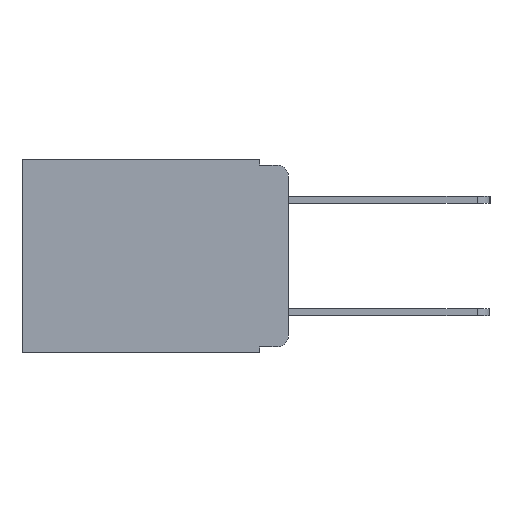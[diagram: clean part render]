
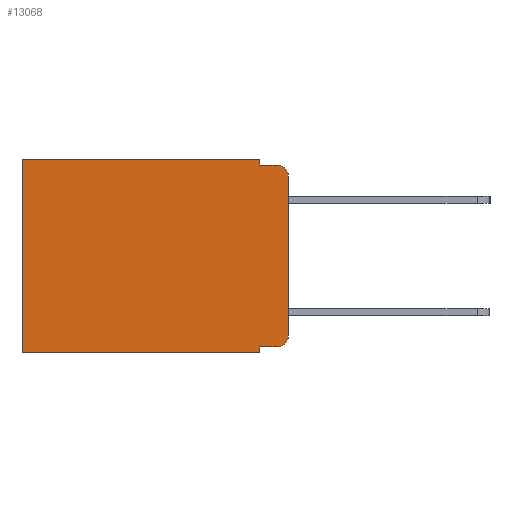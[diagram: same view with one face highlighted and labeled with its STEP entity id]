
A CAD part, left-side view. The second image highlights one B-rep face of the part: STEP entity #13068.
In plain terms, the highlighted planar face has unit normal (-1, 0, 0).
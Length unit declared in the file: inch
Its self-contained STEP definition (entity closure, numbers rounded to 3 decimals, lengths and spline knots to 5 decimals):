
#125 = DIRECTION ( 'NONE',  ( 1., 0., 0. ) ) ;
#245 = EDGE_CURVE ( 'NONE', #4848, #9189, #17565, .T. ) ;
#253 = LINE ( 'NONE', #16846, #16387 ) ;
#279 = EDGE_CURVE ( 'NONE', #9189, #9463, #1811, .T. ) ;
#335 = VERTEX_POINT ( 'NONE', #2833 ) ;
#371 = FACE_OUTER_BOUND ( 'NONE', #6724, .T. ) ;
#1110 = VERTEX_POINT ( 'NONE', #19627 ) ;
#1449 = ORIENTED_EDGE ( 'NONE', *, *, #13762, .F. ) ;
#1811 = CIRCLE ( 'NONE', #2198, 0.02 ) ;
#2198 = AXIS2_PLACEMENT_3D ( 'NONE', #12227, #4207, #6741 ) ;
#2668 = ORIENTED_EDGE ( 'NONE', *, *, #245, .T. ) ;
#2699 = VERTEX_POINT ( 'NONE', #14720 ) ;
#2833 = CARTESIAN_POINT ( 'NONE',  ( 0.298, 0.473, -0.343 ) ) ;
#3286 = EDGE_CURVE ( 'NONE', #2699, #335, #19096, .T. ) ;
#3488 = AXIS2_PLACEMENT_3D ( 'NONE', #6643, #16963, #8152 ) ;
#3841 = CARTESIAN_POINT ( 'NONE',  ( 0.298, 0.051, 0. ) ) ;
#4207 = DIRECTION ( 'NONE',  ( -1., 0., 0. ) ) ;
#4391 = CARTESIAN_POINT ( 'NONE',  ( 0.298, 0., -0.343 ) ) ;
#4655 = VECTOR ( 'NONE', #16420, 39.37008 ) ;
#4704 = CARTESIAN_POINT ( 'NONE',  ( 0.298, 0.051, -0.333 ) ) ;
#4848 = VERTEX_POINT ( 'NONE', #19330 ) ;
#4865 = VERTEX_POINT ( 'NONE', #16603 ) ;
#5349 = ORIENTED_EDGE ( 'NONE', *, *, #16973, .F. ) ;
#5942 = ORIENTED_EDGE ( 'NONE', *, *, #14672, .T. ) ;
#5977 = CARTESIAN_POINT ( 'NONE',  ( 0.298, 0., -0.03 ) ) ;
#6533 = ORIENTED_EDGE ( 'NONE', *, *, #8637, .F. ) ;
#6638 = CARTESIAN_POINT ( 'NONE',  ( 0.298, 0.473, 0. ) ) ;
#6643 = CARTESIAN_POINT ( 'NONE',  ( 0.298, 0.02, -0.03 ) ) ;
#6724 = EDGE_LOOP ( 'NONE', ( #7573, #5942, #1449, #6533, #9975, #18669, #5349, #9994, #2668, #8202 ) ) ;
#6741 = DIRECTION ( 'NONE',  ( 0., 0., -1. ) ) ;
#6802 = CARTESIAN_POINT ( 'NONE',  ( 0.298, 0., -0.313 ) ) ;
#6872 = CARTESIAN_POINT ( 'NONE',  ( 0.298, 0., 0. ) ) ;
#7298 = LINE ( 'NONE', #3841, #14860 ) ;
#7573 = ORIENTED_EDGE ( 'NONE', *, *, #16513, .F. ) ;
#7637 = LINE ( 'NONE', #9679, #15584 ) ;
#8084 = DIRECTION ( 'NONE',  ( 0., 0., -1. ) ) ;
#8144 = VECTOR ( 'NONE', #15929, 39.37008 ) ;
#8152 = DIRECTION ( 'NONE',  ( 0., 0., -1. ) ) ;
#8202 = ORIENTED_EDGE ( 'NONE', *, *, #279, .T. ) ;
#8245 = EDGE_CURVE ( 'NONE', #8499, #2699, #13705, .T. ) ;
#8499 = VERTEX_POINT ( 'NONE', #14156 ) ;
#8637 = EDGE_CURVE ( 'NONE', #8499, #18623, #19236, .T. ) ;
#8804 = DIRECTION ( 'NONE',  ( 0., -1., 0. ) ) ;
#9189 = VERTEX_POINT ( 'NONE', #15847 ) ;
#9463 = VERTEX_POINT ( 'NONE', #6802 ) ;
#9679 = CARTESIAN_POINT ( 'NONE',  ( 0.298, 0.051, -0.01 ) ) ;
#9701 = VECTOR ( 'NONE', #19058, 39.37008 ) ;
#9975 = ORIENTED_EDGE ( 'NONE', *, *, #8245, .T. ) ;
#9994 = ORIENTED_EDGE ( 'NONE', *, *, #17765, .F. ) ;
#10030 = PLANE ( 'NONE',  #14383 ) ;
#11046 = VERTEX_POINT ( 'NONE', #5977 ) ;
#11570 = DIRECTION ( 'NONE',  ( 0., 0., -1. ) ) ;
#12227 = CARTESIAN_POINT ( 'NONE',  ( 0.298, 0.02, -0.313 ) ) ;
#12428 = LINE ( 'NONE', #4391, #4655 ) ;
#13068 = ADVANCED_FACE ( 'NONE', ( #371 ), #10030, .F. ) ;
#13705 = LINE ( 'NONE', #17681, #9701 ) ;
#13762 = EDGE_CURVE ( 'NONE', #18623, #1110, #7637, .T. ) ;
#14156 = CARTESIAN_POINT ( 'NONE',  ( 0.298, 0.051, 0. ) ) ;
#14383 = AXIS2_PLACEMENT_3D ( 'NONE', #6872, #125, #11570 ) ;
#14558 = CARTESIAN_POINT ( 'NONE',  ( 0.298, 0.051, 0. ) ) ;
#14672 = EDGE_CURVE ( 'NONE', #11046, #1110, #15770, .T. ) ;
#14720 = CARTESIAN_POINT ( 'NONE',  ( 0.298, 0.473, 0. ) ) ;
#14860 = VECTOR ( 'NONE', #15985, 39.37008 ) ;
#15457 = VECTOR ( 'NONE', #15573, 39.37008 ) ;
#15573 = DIRECTION ( 'NONE',  ( 0., 0., -1. ) ) ;
#15584 = VECTOR ( 'NONE', #19594, 39.37008 ) ;
#15770 = CIRCLE ( 'NONE', #3488, 0.02 ) ;
#15847 = CARTESIAN_POINT ( 'NONE',  ( 0.298, 0.02, -0.333 ) ) ;
#15929 = DIRECTION ( 'NONE',  ( 0., 0., -1. ) ) ;
#15985 = DIRECTION ( 'NONE',  ( 0., 0., -1. ) ) ;
#16387 = VECTOR ( 'NONE', #8084, 39.37008 ) ;
#16420 = DIRECTION ( 'NONE',  ( 0., 1., 0. ) ) ;
#16513 = EDGE_CURVE ( 'NONE', #11046, #9463, #253, .T. ) ;
#16603 = CARTESIAN_POINT ( 'NONE',  ( 0.298, 0.051, -0.343 ) ) ;
#16846 = CARTESIAN_POINT ( 'NONE',  ( 0.298, 0., 0. ) ) ;
#16963 = DIRECTION ( 'NONE',  ( -1., 0., 0. ) ) ;
#16973 = EDGE_CURVE ( 'NONE', #4865, #335, #12428, .T. ) ;
#17565 = LINE ( 'NONE', #4704, #18026 ) ;
#17681 = CARTESIAN_POINT ( 'NONE',  ( 0.298, 0., 0. ) ) ;
#17765 = EDGE_CURVE ( 'NONE', #4848, #4865, #7298, .T. ) ;
#18026 = VECTOR ( 'NONE', #8804, 39.37008 ) ;
#18313 = CARTESIAN_POINT ( 'NONE',  ( 0.298, 0.051, -0.01 ) ) ;
#18623 = VERTEX_POINT ( 'NONE', #18313 ) ;
#18669 = ORIENTED_EDGE ( 'NONE', *, *, #3286, .T. ) ;
#19058 = DIRECTION ( 'NONE',  ( 0., 1., 0. ) ) ;
#19096 = LINE ( 'NONE', #6638, #15457 ) ;
#19236 = LINE ( 'NONE', #14558, #8144 ) ;
#19330 = CARTESIAN_POINT ( 'NONE',  ( 0.298, 0.051, -0.333 ) ) ;
#19594 = DIRECTION ( 'NONE',  ( 0., -1., 0. ) ) ;
#19627 = CARTESIAN_POINT ( 'NONE',  ( 0.298, 0.02, -0.01 ) ) ;
